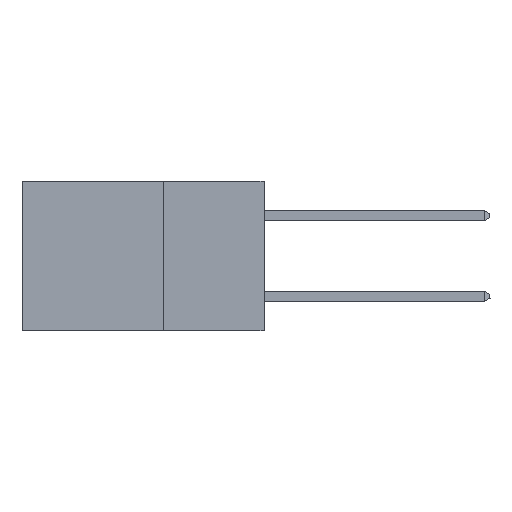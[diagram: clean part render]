
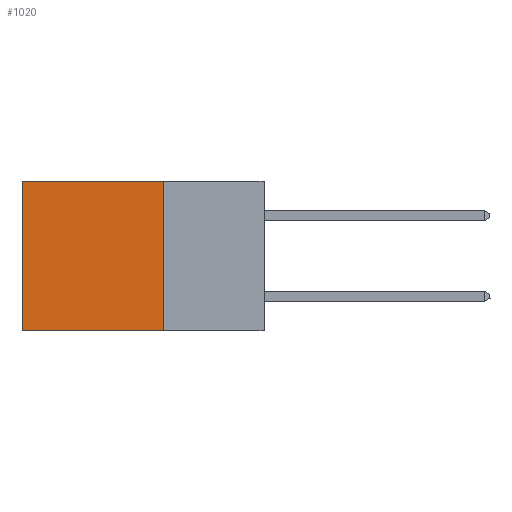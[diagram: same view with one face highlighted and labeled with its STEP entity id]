
A CAD part, left-side view. The second image highlights one B-rep face of the part: STEP entity #1020.
In plain terms, the highlighted planar face has unit normal (-1, 0, 0).
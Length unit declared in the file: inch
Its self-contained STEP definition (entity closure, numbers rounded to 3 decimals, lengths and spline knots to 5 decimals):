
#1005 = ORIENTED_EDGE ( 'NONE', *, *, #3180, .F. ) ;
#1020 = ADVANCED_FACE ( 'NONE', ( #11296 ), #1719, .F. ) ;
#1719 = PLANE ( 'NONE',  #12631 ) ;
#2626 = DIRECTION ( 'NONE',  ( 0., 0., -1. ) ) ;
#2853 = CARTESIAN_POINT ( 'NONE',  ( 0.2615, 0.6, -0.37 ) ) ;
#3180 = EDGE_CURVE ( 'NONE', #23731, #15368, #16505, .T. ) ;
#3515 = VECTOR ( 'NONE', #2626, 39.37008 ) ;
#5034 = LINE ( 'NONE', #2853, #15755 ) ;
#5052 = DIRECTION ( 'NONE',  ( 0., 0., -1. ) ) ;
#5302 = DIRECTION ( 'NONE',  ( 1., 0., 0. ) ) ;
#7437 = CARTESIAN_POINT ( 'NONE',  ( 0.2615, 0.6, -0.37 ) ) ;
#8136 = CARTESIAN_POINT ( 'NONE',  ( 0.2615, 0.25, -0.37 ) ) ;
#9500 = DIRECTION ( 'NONE',  ( 0., 0., -1. ) ) ;
#9674 = CARTESIAN_POINT ( 'NONE',  ( 0.2615, 0.25, 0. ) ) ;
#11296 = FACE_OUTER_BOUND ( 'NONE', #13852, .T. ) ;
#11944 = LINE ( 'NONE', #19998, #27418 ) ;
#12631 = AXIS2_PLACEMENT_3D ( 'NONE', #8136, #5302, #9500 ) ;
#13852 = EDGE_LOOP ( 'NONE', ( #16021, #1005, #15253, #14838 ) ) ;
#13911 = EDGE_CURVE ( 'NONE', #20751, #15368, #5034, .T. ) ;
#14098 = CARTESIAN_POINT ( 'NONE',  ( 0.2615, 0.25, -0.37 ) ) ;
#14838 = ORIENTED_EDGE ( 'NONE', *, *, #25002, .T. ) ;
#15253 = ORIENTED_EDGE ( 'NONE', *, *, #26878, .F. ) ;
#15368 = VERTEX_POINT ( 'NONE', #7437 ) ;
#15755 = VECTOR ( 'NONE', #5052, 39.37008 ) ;
#16021 = ORIENTED_EDGE ( 'NONE', *, *, #13911, .T. ) ;
#16505 = LINE ( 'NONE', #14098, #27005 ) ;
#19825 = CARTESIAN_POINT ( 'NONE',  ( 0.2615, 0.25, -0.37 ) ) ;
#19998 = CARTESIAN_POINT ( 'NONE',  ( 0.2615, 0.25, 0. ) ) ;
#20377 = DIRECTION ( 'NONE',  ( 0., 1., 0. ) ) ;
#20751 = VERTEX_POINT ( 'NONE', #21360 ) ;
#21239 = LINE ( 'NONE', #21758, #3515 ) ;
#21360 = CARTESIAN_POINT ( 'NONE',  ( 0.2615, 0.6, 0. ) ) ;
#21758 = CARTESIAN_POINT ( 'NONE',  ( 0.2615, 0.25, -0.37 ) ) ;
#23731 = VERTEX_POINT ( 'NONE', #19825 ) ;
#25002 = EDGE_CURVE ( 'NONE', #27158, #20751, #11944, .T. ) ;
#26318 = DIRECTION ( 'NONE',  ( 0., 1., 0. ) ) ;
#26878 = EDGE_CURVE ( 'NONE', #27158, #23731, #21239, .T. ) ;
#27005 = VECTOR ( 'NONE', #20377, 39.37008 ) ;
#27158 = VERTEX_POINT ( 'NONE', #9674 ) ;
#27418 = VECTOR ( 'NONE', #26318, 39.37008 ) ;
